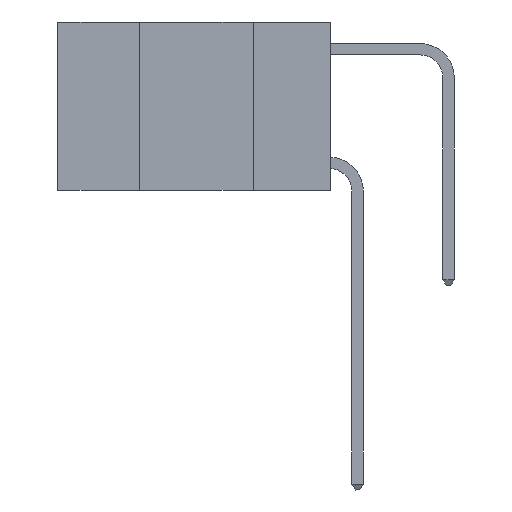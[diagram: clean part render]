
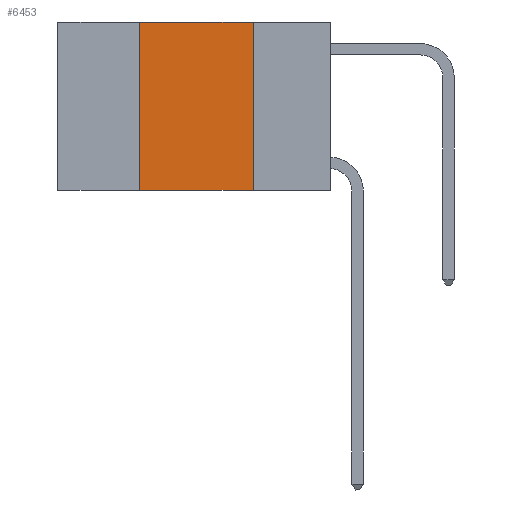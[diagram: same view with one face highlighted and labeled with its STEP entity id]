
A CAD part, left-side view. The second image highlights one B-rep face of the part: STEP entity #6453.
In plain terms, the highlighted planar face has unit normal (-1, 0, 0).
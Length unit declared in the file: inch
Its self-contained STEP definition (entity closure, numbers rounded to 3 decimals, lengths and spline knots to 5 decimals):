
#512 = DIRECTION ( 'NONE',  ( 0., 0., 1. ) ) ;
#641 = AXIS2_PLACEMENT_3D ( 'NONE', #3095, #3209, #6673 ) ;
#646 = DIRECTION ( 'NONE',  ( 0., -1., 0. ) ) ;
#661 = FACE_OUTER_BOUND ( 'NONE', #6053, .T. ) ;
#1207 = ORIENTED_EDGE ( 'NONE', *, *, #9569, .F. ) ;
#1467 = LINE ( 'NONE', #3243, #5886 ) ;
#1513 = CARTESIAN_POINT ( 'NONE',  ( 0., 0.6, 0. ) ) ;
#2358 = VECTOR ( 'NONE', #10466, 39.37008 ) ;
#3055 = CARTESIAN_POINT ( 'NONE',  ( 0., 0.42, 0. ) ) ;
#3095 = CARTESIAN_POINT ( 'NONE',  ( 0., 0.6, 0. ) ) ;
#3209 = DIRECTION ( 'NONE',  ( 1., 0., 0. ) ) ;
#3243 = CARTESIAN_POINT ( 'NONE',  ( 0., 0.6, -0.37 ) ) ;
#3684 = EDGE_CURVE ( 'NONE', #8615, #9266, #9470, .T. ) ;
#4016 = EDGE_CURVE ( 'NONE', #6753, #6559, #1467, .T. ) ;
#4067 = DIRECTION ( 'NONE',  ( 0., 0., -1. ) ) ;
#4396 = VECTOR ( 'NONE', #4067, 39.37008 ) ;
#5109 = CARTESIAN_POINT ( 'NONE',  ( 0., 0.42, -0.37 ) ) ;
#5579 = LINE ( 'NONE', #3055, #7787 ) ;
#5680 = ORIENTED_EDGE ( 'NONE', *, *, #3684, .F. ) ;
#5886 = VECTOR ( 'NONE', #646, 39.37008 ) ;
#6053 = EDGE_LOOP ( 'NONE', ( #11103, #5680, #1207, #7552 ) ) ;
#6453 = ADVANCED_FACE ( 'NONE', ( #661 ), #8637, .F. ) ;
#6559 = VERTEX_POINT ( 'NONE', #11144 ) ;
#6673 = DIRECTION ( 'NONE',  ( 0., 0., -1. ) ) ;
#6753 = VERTEX_POINT ( 'NONE', #5109 ) ;
#7552 = ORIENTED_EDGE ( 'NONE', *, *, #4016, .T. ) ;
#7585 = CARTESIAN_POINT ( 'NONE',  ( 0., 0.42, 0. ) ) ;
#7787 = VECTOR ( 'NONE', #512, 39.37008 ) ;
#7848 = LINE ( 'NONE', #8468, #4396 ) ;
#8019 = CARTESIAN_POINT ( 'NONE',  ( 0., 0.17, 0. ) ) ;
#8468 = CARTESIAN_POINT ( 'NONE',  ( 0., 0.17, 0. ) ) ;
#8615 = VERTEX_POINT ( 'NONE', #7585 ) ;
#8637 = PLANE ( 'NONE',  #641 ) ;
#9168 = EDGE_CURVE ( 'NONE', #9266, #6559, #7848, .T. ) ;
#9266 = VERTEX_POINT ( 'NONE', #8019 ) ;
#9470 = LINE ( 'NONE', #1513, #2358 ) ;
#9569 = EDGE_CURVE ( 'NONE', #6753, #8615, #5579, .T. ) ;
#10466 = DIRECTION ( 'NONE',  ( 0., -1., 0. ) ) ;
#11103 = ORIENTED_EDGE ( 'NONE', *, *, #9168, .F. ) ;
#11144 = CARTESIAN_POINT ( 'NONE',  ( 0., 0.17, -0.37 ) ) ;
